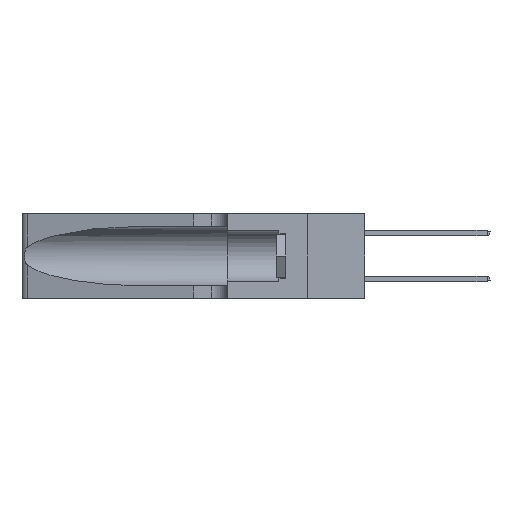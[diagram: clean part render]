
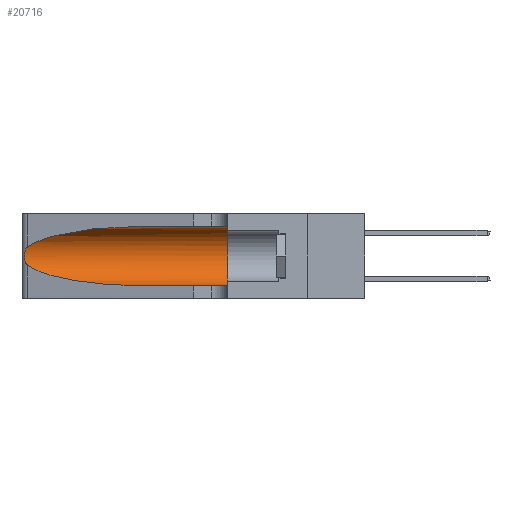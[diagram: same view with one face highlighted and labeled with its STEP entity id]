
A CAD part, left-side view. The second image highlights one B-rep face of the part: STEP entity #20716.
In plain terms, the highlighted cylindrical face has radius 3.308 mm (diameter 6.617 mm), a partial arc.
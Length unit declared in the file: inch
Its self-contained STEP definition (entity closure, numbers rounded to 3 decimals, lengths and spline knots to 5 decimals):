
#890 = CARTESIAN_POINT ( 'NONE',  ( 0.26075, 1.23896, 0.19203 ) ) ;
#1021 = CYLINDRICAL_SURFACE ( 'NONE', #23298, 0.13025 ) ;
#1197 = LINE ( 'NONE', #21923, #25882 ) ;
#2132 = CARTESIAN_POINT ( 'NONE',  ( 0.2373, 1.15595, 0.08982 ) ) ;
#3785 = CARTESIAN_POINT ( 'NONE',  ( 0.26075, 1.23896, 0.178 ) ) ;
#3953 = CARTESIAN_POINT ( 'NONE',  ( 0.25487, 1.22718, 0.22369 ) ) ;
#4528 = CARTESIAN_POINT ( 'NONE',  ( 0.1305, 0.35, 0.31525 ) ) ;
#4692 = VECTOR ( 'NONE', #18785, 39.37008 ) ;
#5591 = EDGE_CURVE ( 'NONE', #19043, #21809, #8301, .T. ) ;
#5674 = ORIENTED_EDGE ( 'NONE', *, *, #35371, .T. ) ;
#5707 = B_SPLINE_CURVE_WITH_KNOTS ( 'NONE', 3,
 ( #34972, #23564, #12332, #35222, #32336, #15158, #890, #3785, #23821, #20455, #21451, #15680, #9708, #18301 ),
 .UNSPECIFIED., .F., .F.,
 ( 4, 2, 2, 2, 2, 2, 4 ),
 ( 0., 0.00027, 0.00053, 0.00107, 0.0016, 0.00187, 0.00214 ),
 .UNSPECIFIED. ) ;
#8203 = CARTESIAN_POINT ( 'NONE',  ( 0.1305, 0.72297, 0.31525 ) ) ;
#8301 = LINE ( 'NONE', #10447, #4692 ) ;
#9708 = CARTESIAN_POINT ( 'NONE',  ( 0.25555, 1.22993, 0.14849 ) ) ;
#10028 = FACE_OUTER_BOUND ( 'NONE', #10804, .T. ) ;
#10447 = CARTESIAN_POINT ( 'NONE',  ( 0.1305, 1.61858, 0.05475 ) ) ;
#10804 = EDGE_LOOP ( 'NONE', ( #15585, #30790, #5674, #27150, #13444, #24781 ) ) ;
#11790 = DIRECTION ( 'NONE',  ( 0., 0., -1. ) ) ;
#12332 = CARTESIAN_POINT ( 'NONE',  ( 0.25639, 1.23184, 0.21858 ) ) ;
#13444 = ORIENTED_EDGE ( 'NONE', *, *, #31092, .F. ) ;
#13952 = CARTESIAN_POINT ( 'NONE',  ( 0.2373, 1.15595, 0.28018 ) ) ;
#14818 = VERTEX_POINT ( 'NONE', #4528 ) ;
#14992 = CARTESIAN_POINT ( 'NONE',  ( 0.1305, 1.61858, 0.185 ) ) ;
#15158 = CARTESIAN_POINT ( 'NONE',  ( 0.26018, 1.23835, 0.19895 ) ) ;
#15585 = ORIENTED_EDGE ( 'NONE', *, *, #26285, .T. ) ;
#15680 = CARTESIAN_POINT ( 'NONE',  ( 0.25639, 1.23186, 0.15144 ) ) ;
#16810 = CARTESIAN_POINT ( 'NONE',  ( 0.25487, 1.22718, 0.14631 ) ) ;
#17593 = CARTESIAN_POINT ( 'NONE',  ( 0.1305, 0.35, 0.185 ) ) ;
#18262 = AXIS2_PLACEMENT_3D ( 'NONE', #17593, #31991, #26643 ) ;
#18301 = CARTESIAN_POINT ( 'NONE',  ( 0.25487, 1.22718, 0.14631 ) ) ;
#18639 = VERTEX_POINT ( 'NONE', #22283 ) ;
#18672 = EDGE_CURVE ( 'NONE', #18639, #14818, #1197, .T. ) ;
#18785 = DIRECTION ( 'NONE',  ( 0., -1., 0. ) ) ;
#19043 = VERTEX_POINT ( 'NONE', #29938 ) ;
#20455 = CARTESIAN_POINT ( 'NONE',  ( 0.25856, 1.23593, 0.16098 ) ) ;
#20716 = ADVANCED_FACE ( 'NONE', ( #10028 ), #1021, .F. ) ;
#21451 = CARTESIAN_POINT ( 'NONE',  ( 0.25789, 1.23486, 0.15765 ) ) ;
#21809 = VERTEX_POINT ( 'NONE', #34345 ) ;
#21923 = CARTESIAN_POINT ( 'NONE',  ( 0.1305, 1.61858, 0.31525 ) ) ;
#22283 = CARTESIAN_POINT ( 'NONE',  ( 0.1305, 0.72297, 0.31525 ) ) ;
#23298 = AXIS2_PLACEMENT_3D ( 'NONE', #14992, #32283, #11790 ) ;
#23564 = CARTESIAN_POINT ( 'NONE',  ( 0.25555, 1.22994, 0.2215 ) ) ;
#23821 = CARTESIAN_POINT ( 'NONE',  ( 0.26017, 1.23833, 0.17102 ) ) ;
#24071 =( BOUNDED_CURVE ( )  B_SPLINE_CURVE ( 3, ( #16810, #2132, #28362, #28110 ),
 .UNSPECIFIED., .F., .T. ) 
 B_SPLINE_CURVE_WITH_KNOTS ( ( 4, 4 ),
 ( 3.44316, 4.71239 ),
 .UNSPECIFIED. ) 
 CURVE ( )  GEOMETRIC_REPRESENTATION_ITEM ( )  RATIONAL_B_SPLINE_CURVE ( ( 1., 0.87, 0.87, 1. ) ) 
 REPRESENTATION_ITEM ( '' )  );
#24781 = ORIENTED_EDGE ( 'NONE', *, *, #18672, .F. ) ;
#25882 = VECTOR ( 'NONE', #30705, 39.37008 ) ;
#26285 = EDGE_CURVE ( 'NONE', #18639, #34360, #34155, .T. ) ;
#26643 = DIRECTION ( 'NONE',  ( 0., 0., 1. ) ) ;
#27150 = ORIENTED_EDGE ( 'NONE', *, *, #5591, .T. ) ;
#27880 = CARTESIAN_POINT ( 'NONE',  ( 0.25487, 1.22718, 0.22369 ) ) ;
#28110 = CARTESIAN_POINT ( 'NONE',  ( 0.1305, 0.72297, 0.05475 ) ) ;
#28252 = CARTESIAN_POINT ( 'NONE',  ( 0.18966, 0.96281, 0.31525 ) ) ;
#28362 = CARTESIAN_POINT ( 'NONE',  ( 0.18966, 0.96281, 0.05475 ) ) ;
#29938 = CARTESIAN_POINT ( 'NONE',  ( 0.1305, 0.72297, 0.05475 ) ) ;
#30705 = DIRECTION ( 'NONE',  ( 0., -1., 0. ) ) ;
#30790 = ORIENTED_EDGE ( 'NONE', *, *, #33153, .T. ) ;
#31092 = EDGE_CURVE ( 'NONE', #14818, #21809, #35439, .T. ) ;
#31991 = DIRECTION ( 'NONE',  ( 0., 1., 0. ) ) ;
#32283 = DIRECTION ( 'NONE',  ( 0., -1., 0. ) ) ;
#32336 = CARTESIAN_POINT ( 'NONE',  ( 0.25854, 1.2359, 0.20912 ) ) ;
#32917 = CARTESIAN_POINT ( 'NONE',  ( 0.25487, 1.22718, 0.14631 ) ) ;
#33153 = EDGE_CURVE ( 'NONE', #34360, #35707, #5707, .T. ) ;
#34155 =( BOUNDED_CURVE ( )  B_SPLINE_CURVE ( 3, ( #8203, #28252, #13952, #27880 ),
 .UNSPECIFIED., .F., .F. ) 
 B_SPLINE_CURVE_WITH_KNOTS ( ( 4, 4 ),
 ( 1.5708, 2.84003 ),
 .UNSPECIFIED. ) 
 CURVE ( )  GEOMETRIC_REPRESENTATION_ITEM ( )  RATIONAL_B_SPLINE_CURVE ( ( 1., 0.87, 0.87, 1. ) ) 
 REPRESENTATION_ITEM ( '' )  );
#34345 = CARTESIAN_POINT ( 'NONE',  ( 0.1305, 0.35, 0.05475 ) ) ;
#34360 = VERTEX_POINT ( 'NONE', #3953 ) ;
#34972 = CARTESIAN_POINT ( 'NONE',  ( 0.25487, 1.22718, 0.22369 ) ) ;
#35222 = CARTESIAN_POINT ( 'NONE',  ( 0.25787, 1.23484, 0.2124 ) ) ;
#35371 = EDGE_CURVE ( 'NONE', #35707, #19043, #24071, .T. ) ;
#35439 = CIRCLE ( 'NONE', #18262, 0.13025 ) ;
#35707 = VERTEX_POINT ( 'NONE', #32917 ) ;
